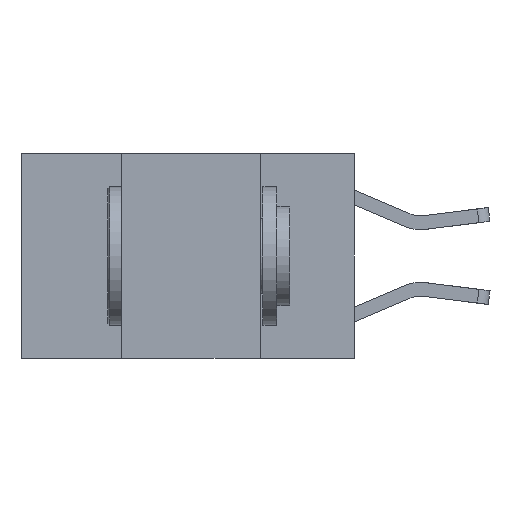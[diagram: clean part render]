
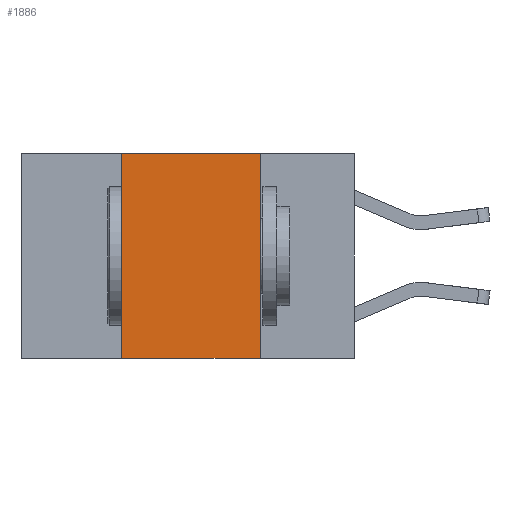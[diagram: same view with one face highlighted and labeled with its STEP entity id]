
A CAD part, left-side view. The second image highlights one B-rep face of the part: STEP entity #1886.
In plain terms, the highlighted planar face has unit normal (-1, 0, 0).
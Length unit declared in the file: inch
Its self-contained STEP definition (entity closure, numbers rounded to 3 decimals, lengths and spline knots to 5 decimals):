
#768 = VERTEX_POINT ( 'NONE', #10646 ) ;
#888 = ORIENTED_EDGE ( 'NONE', *, *, #5543, .F. ) ;
#904 = DIRECTION ( 'NONE',  ( 0., 0., -1. ) ) ;
#907 = DIRECTION ( 'NONE',  ( 1., 0., 0. ) ) ;
#964 = CARTESIAN_POINT ( 'NONE',  ( 0., 0.6, 0. ) ) ;
#979 = DIRECTION ( 'NONE',  ( 0., 0., 1. ) ) ;
#1020 = PLANE ( 'NONE',  #10862 ) ;
#1042 = DIRECTION ( 'NONE',  ( 0., -1., 0. ) ) ;
#1064 = LINE ( 'NONE', #9607, #10953 ) ;
#1127 = CARTESIAN_POINT ( 'NONE',  ( 0., 0.17, 0. ) ) ;
#1375 = VECTOR ( 'NONE', #979, 39.37008 ) ;
#1886 = ADVANCED_FACE ( 'NONE', ( #10682 ), #1020, .F. ) ;
#2554 = VERTEX_POINT ( 'NONE', #1127 ) ;
#2581 = ORIENTED_EDGE ( 'NONE', *, *, #4555, .F. ) ;
#2959 = DIRECTION ( 'NONE',  ( 0., 0., -1. ) ) ;
#3270 = CARTESIAN_POINT ( 'NONE',  ( 0., 0.42, -0.37 ) ) ;
#3462 = CARTESIAN_POINT ( 'NONE',  ( 0., 0.6, 0. ) ) ;
#4005 = LINE ( 'NONE', #4868, #1375 ) ;
#4341 = DIRECTION ( 'NONE',  ( 0., -1., 0. ) ) ;
#4555 = EDGE_CURVE ( 'NONE', #9906, #2554, #7773, .T. ) ;
#4745 = CARTESIAN_POINT ( 'NONE',  ( 0., 0.42, 0. ) ) ;
#4868 = CARTESIAN_POINT ( 'NONE',  ( 0., 0.42, 0. ) ) ;
#5527 = EDGE_CURVE ( 'NONE', #2554, #768, #9352, .T. ) ;
#5543 = EDGE_CURVE ( 'NONE', #11441, #9906, #4005, .T. ) ;
#5561 = EDGE_CURVE ( 'NONE', #11441, #768, #1064, .T. ) ;
#5772 = EDGE_LOOP ( 'NONE', ( #12387, #2581, #888, #11981 ) ) ;
#7773 = LINE ( 'NONE', #3462, #12183 ) ;
#9063 = VECTOR ( 'NONE', #2959, 39.37008 ) ;
#9352 = LINE ( 'NONE', #11438, #9063 ) ;
#9607 = CARTESIAN_POINT ( 'NONE',  ( 0., 0.6, -0.37 ) ) ;
#9906 = VERTEX_POINT ( 'NONE', #4745 ) ;
#10646 = CARTESIAN_POINT ( 'NONE',  ( 0., 0.17, -0.37 ) ) ;
#10682 = FACE_OUTER_BOUND ( 'NONE', #5772, .T. ) ;
#10862 = AXIS2_PLACEMENT_3D ( 'NONE', #964, #907, #904 ) ;
#10953 = VECTOR ( 'NONE', #1042, 39.37008 ) ;
#11438 = CARTESIAN_POINT ( 'NONE',  ( 0., 0.17, 0. ) ) ;
#11441 = VERTEX_POINT ( 'NONE', #3270 ) ;
#11981 = ORIENTED_EDGE ( 'NONE', *, *, #5561, .T. ) ;
#12183 = VECTOR ( 'NONE', #4341, 39.37008 ) ;
#12387 = ORIENTED_EDGE ( 'NONE', *, *, #5527, .F. ) ;
